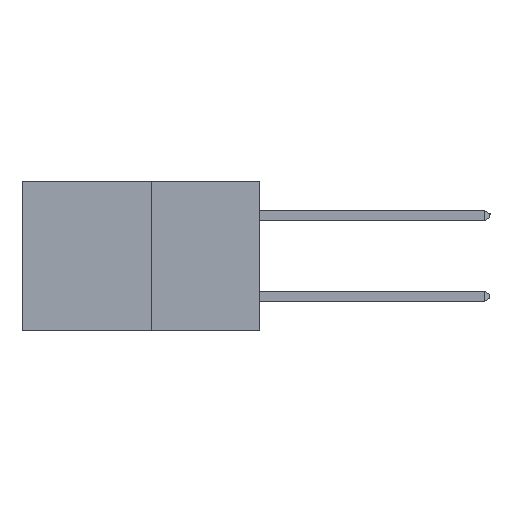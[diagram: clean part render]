
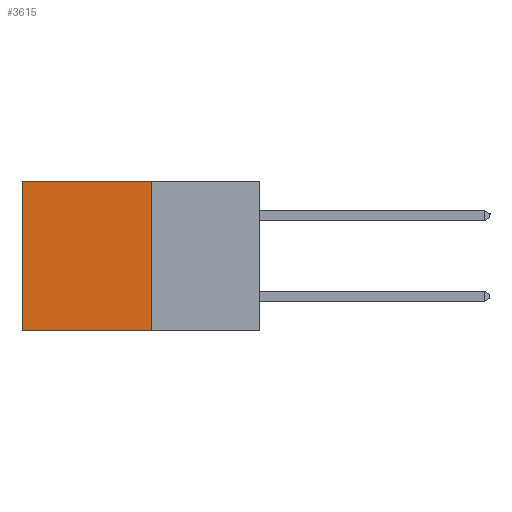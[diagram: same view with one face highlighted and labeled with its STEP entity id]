
A CAD part, left-side view. The second image highlights one B-rep face of the part: STEP entity #3615.
In plain terms, the highlighted planar face has unit normal (-1, 0, 0).
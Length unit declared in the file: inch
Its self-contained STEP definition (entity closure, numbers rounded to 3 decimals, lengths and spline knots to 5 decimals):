
#264 = VECTOR ( 'NONE', #2245, 39.37008 ) ;
#424 = ORIENTED_EDGE ( 'NONE', *, *, #2278, .F. ) ;
#814 = CARTESIAN_POINT ( 'NONE',  ( 0.277, 0.27, -0.37 ) ) ;
#969 = LINE ( 'NONE', #6866, #8732 ) ;
#1015 = VERTEX_POINT ( 'NONE', #6859 ) ;
#1701 = LINE ( 'NONE', #2846, #9196 ) ;
#1753 = DIRECTION ( 'NONE',  ( 0., 0., -1. ) ) ;
#1889 = EDGE_CURVE ( 'NONE', #5896, #2668, #969, .T. ) ;
#2055 = AXIS2_PLACEMENT_3D ( 'NONE', #8051, #9113, #1753 ) ;
#2245 = DIRECTION ( 'NONE',  ( 0., 0., -1. ) ) ;
#2278 = EDGE_CURVE ( 'NONE', #5896, #6040, #9289, .T. ) ;
#2439 = ORIENTED_EDGE ( 'NONE', *, *, #1889, .T. ) ;
#2457 = DIRECTION ( 'NONE',  ( 0., 0., -1. ) ) ;
#2668 = VERTEX_POINT ( 'NONE', #6814 ) ;
#2811 = EDGE_LOOP ( 'NONE', ( #4183, #8036, #424, #2439 ) ) ;
#2846 = CARTESIAN_POINT ( 'NONE',  ( 0.277, 0.59, -0.37 ) ) ;
#3364 = CARTESIAN_POINT ( 'NONE',  ( 0.277, 0.27, 0. ) ) ;
#3615 = ADVANCED_FACE ( 'NONE', ( #3631 ), #8049, .F. ) ;
#3631 = FACE_OUTER_BOUND ( 'NONE', #2811, .T. ) ;
#3810 = DIRECTION ( 'NONE',  ( 0., 1., 0. ) ) ;
#4083 = CARTESIAN_POINT ( 'NONE',  ( 0.277, 0.27, -0.37 ) ) ;
#4183 = ORIENTED_EDGE ( 'NONE', *, *, #6985, .T. ) ;
#4285 = CARTESIAN_POINT ( 'NONE',  ( 0.277, 0.27, -0.37 ) ) ;
#4866 = LINE ( 'NONE', #4083, #8223 ) ;
#5896 = VERTEX_POINT ( 'NONE', #3364 ) ;
#6040 = VERTEX_POINT ( 'NONE', #814 ) ;
#6814 = CARTESIAN_POINT ( 'NONE',  ( 0.277, 0.59, 0. ) ) ;
#6852 = DIRECTION ( 'NONE',  ( 0., 1., 0. ) ) ;
#6859 = CARTESIAN_POINT ( 'NONE',  ( 0.277, 0.59, -0.37 ) ) ;
#6866 = CARTESIAN_POINT ( 'NONE',  ( 0.277, 0.27, 0. ) ) ;
#6885 = EDGE_CURVE ( 'NONE', #6040, #1015, #4866, .T. ) ;
#6985 = EDGE_CURVE ( 'NONE', #2668, #1015, #1701, .T. ) ;
#8036 = ORIENTED_EDGE ( 'NONE', *, *, #6885, .F. ) ;
#8049 = PLANE ( 'NONE',  #2055 ) ;
#8051 = CARTESIAN_POINT ( 'NONE',  ( 0.277, 0.27, -0.37 ) ) ;
#8223 = VECTOR ( 'NONE', #3810, 39.37008 ) ;
#8732 = VECTOR ( 'NONE', #6852, 39.37008 ) ;
#9113 = DIRECTION ( 'NONE',  ( 1., 0., 0. ) ) ;
#9196 = VECTOR ( 'NONE', #2457, 39.37008 ) ;
#9289 = LINE ( 'NONE', #4285, #264 ) ;
